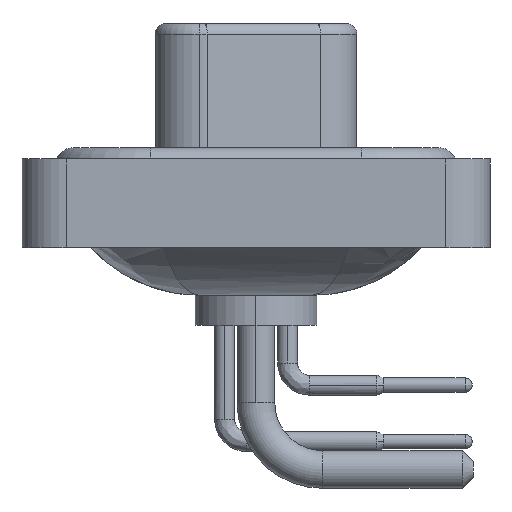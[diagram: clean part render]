
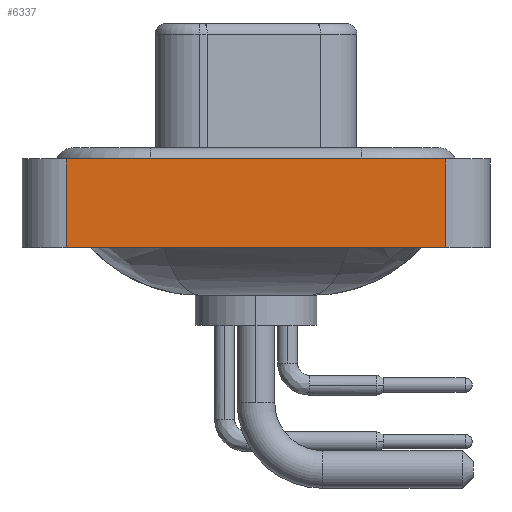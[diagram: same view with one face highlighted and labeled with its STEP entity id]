
A CAD part, left-side view. The second image highlights one B-rep face of the part: STEP entity #6337.
In plain terms, the highlighted planar face has unit normal (-1, 0, 0).
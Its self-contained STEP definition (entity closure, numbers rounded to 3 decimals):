
#449 = PLANE ( 'NONE',  #13670 ) ;
#1509 = VECTOR ( 'NONE', #12244, 1000. ) ;
#4400 = ORIENTED_EDGE ( 'NONE', *, *, #16487, .T. ) ;
#4491 = LINE ( 'NONE', #8491, #24737 ) ;
#4604 = CARTESIAN_POINT ( 'NONE',  ( -7.35, 8.55, -3.6 ) ) ;
#5306 = EDGE_CURVE ( 'NONE', #13772, #24504, #4491, .T. ) ;
#5623 = CARTESIAN_POINT ( 'NONE',  ( -7.35, 8.55, -3.6 ) ) ;
#6337 = ADVANCED_FACE ( 'NONE', ( #21426 ), #449, .T. ) ;
#7267 = LINE ( 'NONE', #5623, #9610 ) ;
#7561 = DIRECTION ( 'NONE',  ( 0., 0., 1. ) ) ;
#7814 = CARTESIAN_POINT ( 'NONE',  ( -7.35, -8.55, 0.4 ) ) ;
#8317 = VECTOR ( 'NONE', #14693, 1000. ) ;
#8491 = CARTESIAN_POINT ( 'NONE',  ( -7.35, -8.55, -3.6 ) ) ;
#8838 = CARTESIAN_POINT ( 'NONE',  ( -7.35, -8.55, -3.6 ) ) ;
#8985 = ORIENTED_EDGE ( 'NONE', *, *, #21087, .F. ) ;
#9565 = ORIENTED_EDGE ( 'NONE', *, *, #15660, .F. ) ;
#9610 = VECTOR ( 'NONE', #7561, 1000. ) ;
#11768 = CARTESIAN_POINT ( 'NONE',  ( -7.35, -8.55, 0.4 ) ) ;
#11834 = LINE ( 'NONE', #7814, #1509 ) ;
#12009 = CARTESIAN_POINT ( 'NONE',  ( -7.35, 8.55, 0.4 ) ) ;
#12194 = LINE ( 'NONE', #22999, #8317 ) ;
#12244 = DIRECTION ( 'NONE',  ( 0., -1., 0. ) ) ;
#13670 = AXIS2_PLACEMENT_3D ( 'NONE', #8838, #26415, #24763 ) ;
#13772 = VERTEX_POINT ( 'NONE', #4604 ) ;
#14693 = DIRECTION ( 'NONE',  ( 0., 0., 1. ) ) ;
#14740 = DIRECTION ( 'NONE',  ( 0., -1., 0. ) ) ;
#15660 = EDGE_CURVE ( 'NONE', #13772, #18768, #7267, .T. ) ;
#16487 = EDGE_CURVE ( 'NONE', #24504, #23236, #12194, .T. ) ;
#18768 = VERTEX_POINT ( 'NONE', #12009 ) ;
#21087 = EDGE_CURVE ( 'NONE', #18768, #23236, #11834, .T. ) ;
#21426 = FACE_OUTER_BOUND ( 'NONE', #27042, .T. ) ;
#22268 = ORIENTED_EDGE ( 'NONE', *, *, #5306, .T. ) ;
#22999 = CARTESIAN_POINT ( 'NONE',  ( -7.35, -8.55, -3.6 ) ) ;
#23236 = VERTEX_POINT ( 'NONE', #11768 ) ;
#24504 = VERTEX_POINT ( 'NONE', #26309 ) ;
#24737 = VECTOR ( 'NONE', #14740, 1000. ) ;
#24763 = DIRECTION ( 'NONE',  ( 0., 0., 1. ) ) ;
#26309 = CARTESIAN_POINT ( 'NONE',  ( -7.35, -8.55, -3.6 ) ) ;
#26415 = DIRECTION ( 'NONE',  ( -1., 0., 0. ) ) ;
#27042 = EDGE_LOOP ( 'NONE', ( #4400, #8985, #9565, #22268 ) ) ;
